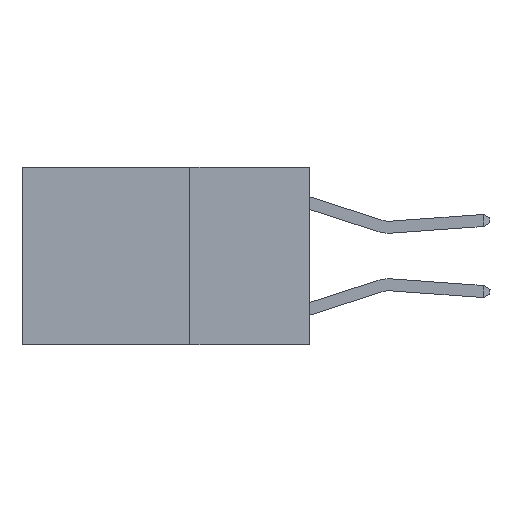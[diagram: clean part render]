
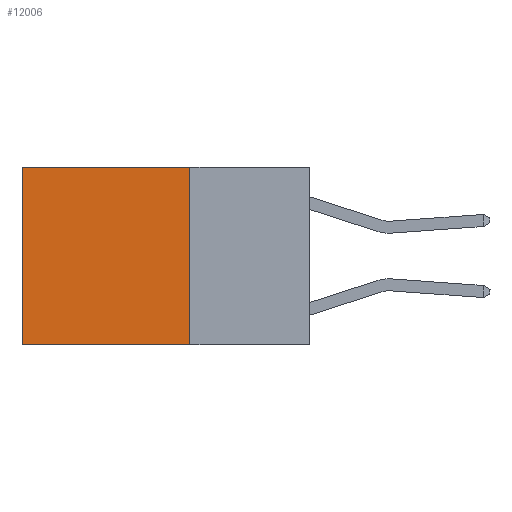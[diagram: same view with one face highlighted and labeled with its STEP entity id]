
A CAD part, left-side view. The second image highlights one B-rep face of the part: STEP entity #12006.
In plain terms, the highlighted planar face has unit normal (-1, 0, 0).
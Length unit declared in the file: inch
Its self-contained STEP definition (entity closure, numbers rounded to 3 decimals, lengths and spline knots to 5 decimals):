
#824 = ORIENTED_EDGE ( 'NONE', *, *, #1600, .T. ) ;
#1600 = EDGE_CURVE ( 'NONE', #27772, #12948, #20678, .T. ) ;
#1861 = EDGE_CURVE ( 'NONE', #6174, #27772, #10154, .T. ) ;
#2729 = FACE_OUTER_BOUND ( 'NONE', #13501, .T. ) ;
#3248 = EDGE_CURVE ( 'NONE', #16466, #12948, #24947, .T. ) ;
#4151 = ORIENTED_EDGE ( 'NONE', *, *, #1861, .T. ) ;
#4373 = VECTOR ( 'NONE', #13697, 39.37008 ) ;
#5017 = CARTESIAN_POINT ( 'NONE',  ( 0.2625, 0.6, 0. ) ) ;
#5121 = CARTESIAN_POINT ( 'NONE',  ( 0.2625, 0.6, 0. ) ) ;
#6174 = VERTEX_POINT ( 'NONE', #8236 ) ;
#7001 = CARTESIAN_POINT ( 'NONE',  ( 0.2625, 0.25, 0. ) ) ;
#7364 = DIRECTION ( 'NONE',  ( 0., 0., -1. ) ) ;
#7768 = DIRECTION ( 'NONE',  ( 1., 0., 0. ) ) ;
#7930 = ORIENTED_EDGE ( 'NONE', *, *, #3248, .F. ) ;
#8046 = DIRECTION ( 'NONE',  ( 0., 0., -1. ) ) ;
#8236 = CARTESIAN_POINT ( 'NONE',  ( 0.2625, 0.25, 0. ) ) ;
#9742 = PLANE ( 'NONE',  #14278 ) ;
#10154 = LINE ( 'NONE', #20366, #4373 ) ;
#10516 = VECTOR ( 'NONE', #18329, 39.37008 ) ;
#12006 = ADVANCED_FACE ( 'NONE', ( #2729 ), #9742, .F. ) ;
#12948 = VERTEX_POINT ( 'NONE', #22166 ) ;
#13501 = EDGE_LOOP ( 'NONE', ( #824, #7930, #16091, #4151 ) ) ;
#13697 = DIRECTION ( 'NONE',  ( 0., 1., 0. ) ) ;
#14278 = AXIS2_PLACEMENT_3D ( 'NONE', #16844, #7768, #8046 ) ;
#14760 = VECTOR ( 'NONE', #7364, 39.37008 ) ;
#15251 = EDGE_CURVE ( 'NONE', #6174, #16466, #23954, .T. ) ;
#15608 = CARTESIAN_POINT ( 'NONE',  ( 0.2625, 0.25, -0.37 ) ) ;
#16091 = ORIENTED_EDGE ( 'NONE', *, *, #15251, .F. ) ;
#16466 = VERTEX_POINT ( 'NONE', #26307 ) ;
#16844 = CARTESIAN_POINT ( 'NONE',  ( 0.2625, 0.25, 0. ) ) ;
#18329 = DIRECTION ( 'NONE',  ( 0., 0., -1. ) ) ;
#20366 = CARTESIAN_POINT ( 'NONE',  ( 0.2625, 0.25, 0. ) ) ;
#20678 = LINE ( 'NONE', #5121, #10516 ) ;
#22166 = CARTESIAN_POINT ( 'NONE',  ( 0.2625, 0.6, -0.37 ) ) ;
#23954 = LINE ( 'NONE', #7001, #14760 ) ;
#24322 = DIRECTION ( 'NONE',  ( 0., 1., 0. ) ) ;
#24947 = LINE ( 'NONE', #15608, #27628 ) ;
#26307 = CARTESIAN_POINT ( 'NONE',  ( 0.2625, 0.25, -0.37 ) ) ;
#27628 = VECTOR ( 'NONE', #24322, 39.37008 ) ;
#27772 = VERTEX_POINT ( 'NONE', #5017 ) ;
